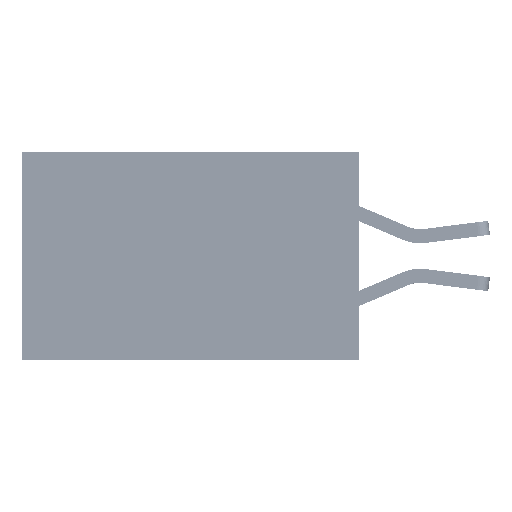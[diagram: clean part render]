
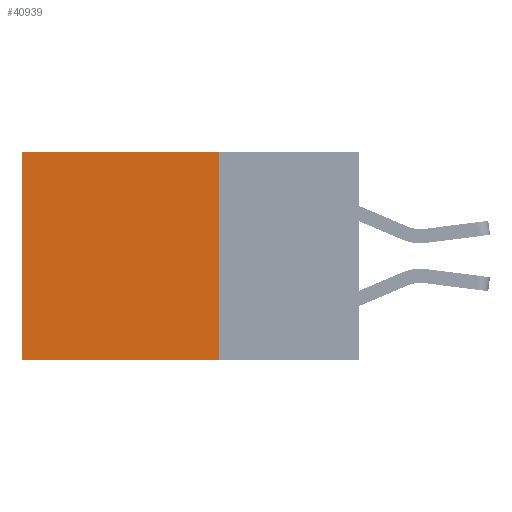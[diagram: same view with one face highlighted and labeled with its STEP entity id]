
A CAD part, left-side view. The second image highlights one B-rep face of the part: STEP entity #40939.
In plain terms, the highlighted planar face has unit normal (-1, 0, 0).
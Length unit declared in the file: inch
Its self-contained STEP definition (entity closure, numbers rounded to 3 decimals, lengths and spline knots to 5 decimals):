
#1982 = CARTESIAN_POINT ( 'NONE',  ( 0.2875, 0.25, -0.37 ) ) ;
#2668 = EDGE_CURVE ( 'NONE', #4470, #31980, #43077, .T. ) ;
#3861 = ORIENTED_EDGE ( 'NONE', *, *, #10639, .T. ) ;
#4027 = CARTESIAN_POINT ( 'NONE',  ( 0.2875, 0.6, 0. ) ) ;
#4470 = VERTEX_POINT ( 'NONE', #1982 ) ;
#4922 = VECTOR ( 'NONE', #6808, 39.37008 ) ;
#5350 = LINE ( 'NONE', #13693, #29533 ) ;
#5576 = CARTESIAN_POINT ( 'NONE',  ( 0.2875, 0.6, -0.37 ) ) ;
#6808 = DIRECTION ( 'NONE',  ( 0., 0., -1. ) ) ;
#8150 = VECTOR ( 'NONE', #10343, 39.37008 ) ;
#9153 = DIRECTION ( 'NONE',  ( 0., 1., 0. ) ) ;
#10343 = DIRECTION ( 'NONE',  ( 0., 0., -1. ) ) ;
#10639 = EDGE_CURVE ( 'NONE', #42638, #31980, #41445, .T. ) ;
#11506 = VERTEX_POINT ( 'NONE', #37025 ) ;
#12736 = CARTESIAN_POINT ( 'NONE',  ( 0.2875, 0.25, 0. ) ) ;
#13557 = AXIS2_PLACEMENT_3D ( 'NONE', #12736, #24350, #24111 ) ;
#13693 = CARTESIAN_POINT ( 'NONE',  ( 0.2875, 0.25, 0. ) ) ;
#15861 = ORIENTED_EDGE ( 'NONE', *, *, #2668, .F. ) ;
#16117 = ORIENTED_EDGE ( 'NONE', *, *, #27931, .F. ) ;
#17162 = EDGE_CURVE ( 'NONE', #11506, #42638, #5350, .T. ) ;
#17500 = DIRECTION ( 'NONE',  ( 0., 1., 0. ) ) ;
#19384 = EDGE_LOOP ( 'NONE', ( #3861, #15861, #16117, #23418 ) ) ;
#22215 = CARTESIAN_POINT ( 'NONE',  ( 0.2875, 0.6, 0. ) ) ;
#22253 = LINE ( 'NONE', #29835, #4922 ) ;
#23418 = ORIENTED_EDGE ( 'NONE', *, *, #17162, .T. ) ;
#24111 = DIRECTION ( 'NONE',  ( 0., 0., -1. ) ) ;
#24350 = DIRECTION ( 'NONE',  ( 1., 0., 0. ) ) ;
#27931 = EDGE_CURVE ( 'NONE', #11506, #4470, #22253, .T. ) ;
#28386 = PLANE ( 'NONE',  #13557 ) ;
#29533 = VECTOR ( 'NONE', #17500, 39.37008 ) ;
#29835 = CARTESIAN_POINT ( 'NONE',  ( 0.2875, 0.25, 0. ) ) ;
#31980 = VERTEX_POINT ( 'NONE', #5576 ) ;
#37025 = CARTESIAN_POINT ( 'NONE',  ( 0.2875, 0.25, 0. ) ) ;
#39761 = CARTESIAN_POINT ( 'NONE',  ( 0.2875, 0.25, -0.37 ) ) ;
#40429 = VECTOR ( 'NONE', #9153, 39.37008 ) ;
#40939 = ADVANCED_FACE ( 'NONE', ( #46202 ), #28386, .F. ) ;
#41445 = LINE ( 'NONE', #22215, #8150 ) ;
#42638 = VERTEX_POINT ( 'NONE', #4027 ) ;
#43077 = LINE ( 'NONE', #39761, #40429 ) ;
#46202 = FACE_OUTER_BOUND ( 'NONE', #19384, .T. ) ;
